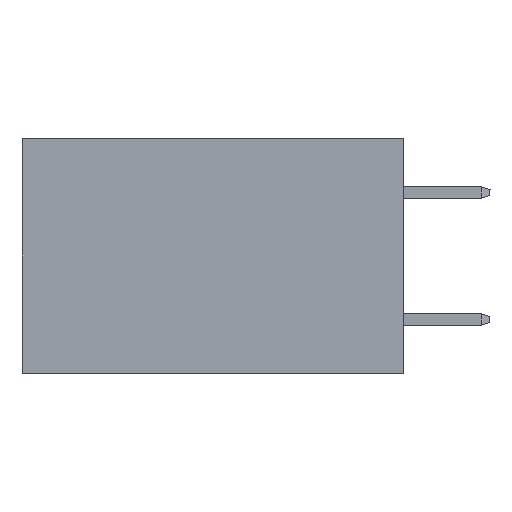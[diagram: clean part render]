
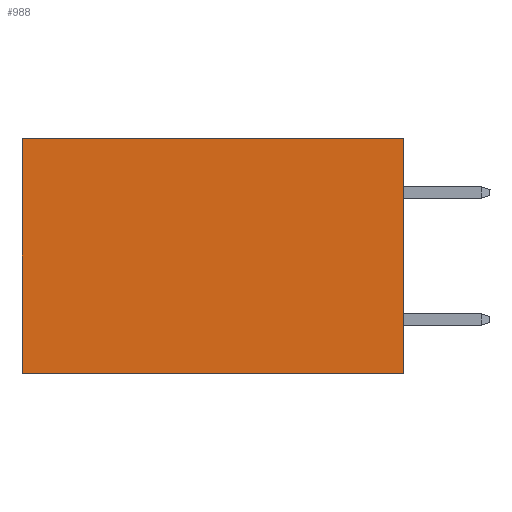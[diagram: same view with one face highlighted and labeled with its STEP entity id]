
A CAD part, left-side view. The second image highlights one B-rep face of the part: STEP entity #988.
In plain terms, the highlighted planar face has unit normal (-1, 0, 0).
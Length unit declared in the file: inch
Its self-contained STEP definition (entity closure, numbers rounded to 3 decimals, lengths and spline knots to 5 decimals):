
#790 = FACE_OUTER_BOUND ( 'NONE', #35023, .T. ) ;
#988 = ADVANCED_FACE ( 'NONE', ( #790 ), #19989, .F. ) ;
#5321 = CARTESIAN_POINT ( 'NONE',  ( 0.2875, 0., 0. ) ) ;
#6086 = EDGE_CURVE ( 'NONE', #14847, #21048, #38689, .T. ) ;
#6734 = EDGE_CURVE ( 'NONE', #33994, #14847, #33572, .T. ) ;
#7358 = CARTESIAN_POINT ( 'NONE',  ( 0.2875, 0., 0. ) ) ;
#7379 = CARTESIAN_POINT ( 'NONE',  ( 0.2875, 0., -0.37 ) ) ;
#9135 = VERTEX_POINT ( 'NONE', #7379 ) ;
#9247 = CARTESIAN_POINT ( 'NONE',  ( 0.2875, 0.6, 0. ) ) ;
#10501 = CARTESIAN_POINT ( 'NONE',  ( 0.2875, 0., 0. ) ) ;
#11807 = VECTOR ( 'NONE', #35459, 39.37008 ) ;
#12578 = DIRECTION ( 'NONE',  ( 0., 1., 0. ) ) ;
#12772 = CARTESIAN_POINT ( 'NONE',  ( 0.2875, 0.6, -0.37 ) ) ;
#12807 = LINE ( 'NONE', #7358, #35456 ) ;
#14590 = DIRECTION ( 'NONE',  ( 0., 1., 0. ) ) ;
#14847 = VERTEX_POINT ( 'NONE', #9247 ) ;
#16569 = DIRECTION ( 'NONE',  ( 1., 0., 0. ) ) ;
#19989 = PLANE ( 'NONE',  #34661 ) ;
#21048 = VERTEX_POINT ( 'NONE', #12772 ) ;
#22782 = ORIENTED_EDGE ( 'NONE', *, *, #33785, .F. ) ;
#24813 = EDGE_CURVE ( 'NONE', #9135, #21048, #37228, .T. ) ;
#25117 = DIRECTION ( 'NONE',  ( 0., 0., -1. ) ) ;
#27359 = VECTOR ( 'NONE', #14590, 39.37008 ) ;
#28126 = CARTESIAN_POINT ( 'NONE',  ( 0.2875, 0., -0.37 ) ) ;
#29300 = DIRECTION ( 'NONE',  ( 0., 0., -1. ) ) ;
#30148 = ORIENTED_EDGE ( 'NONE', *, *, #24813, .F. ) ;
#30350 = CARTESIAN_POINT ( 'NONE',  ( 0.2875, 0., 0. ) ) ;
#31832 = CARTESIAN_POINT ( 'NONE',  ( 0.2875, 0.6, 0. ) ) ;
#32102 = ORIENTED_EDGE ( 'NONE', *, *, #6734, .T. ) ;
#32566 = VECTOR ( 'NONE', #12578, 39.37008 ) ;
#33572 = LINE ( 'NONE', #30350, #27359 ) ;
#33785 = EDGE_CURVE ( 'NONE', #33994, #9135, #12807, .T. ) ;
#33994 = VERTEX_POINT ( 'NONE', #5321 ) ;
#34661 = AXIS2_PLACEMENT_3D ( 'NONE', #10501, #16569, #29300 ) ;
#35023 = EDGE_LOOP ( 'NONE', ( #35323, #30148, #22782, #32102 ) ) ;
#35323 = ORIENTED_EDGE ( 'NONE', *, *, #6086, .T. ) ;
#35456 = VECTOR ( 'NONE', #25117, 39.37008 ) ;
#35459 = DIRECTION ( 'NONE',  ( 0., 0., -1. ) ) ;
#37228 = LINE ( 'NONE', #28126, #32566 ) ;
#38689 = LINE ( 'NONE', #31832, #11807 ) ;
